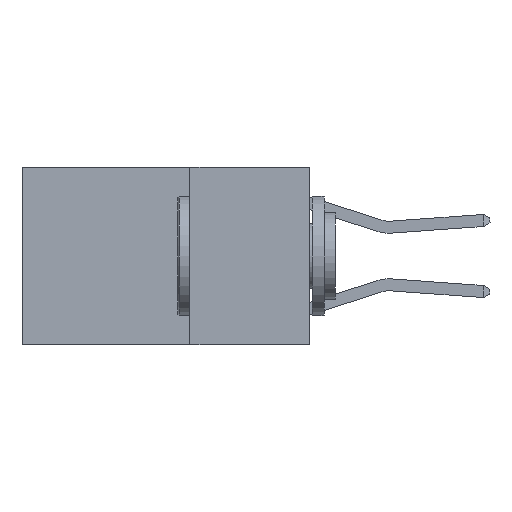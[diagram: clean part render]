
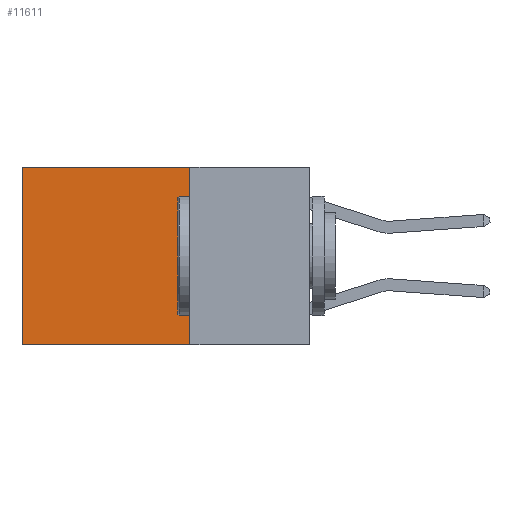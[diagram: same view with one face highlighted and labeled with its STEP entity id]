
A CAD part, left-side view. The second image highlights one B-rep face of the part: STEP entity #11611.
In plain terms, the highlighted planar face has unit normal (-1, 0, 0).
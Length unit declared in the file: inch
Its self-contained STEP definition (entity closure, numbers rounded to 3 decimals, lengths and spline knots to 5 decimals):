
#410 = PLANE ( 'NONE',  #19959 ) ;
#2105 = VERTEX_POINT ( 'NONE', #9692 ) ;
#2933 = DIRECTION ( 'NONE',  ( 0., 0., -1. ) ) ;
#3425 = LINE ( 'NONE', #7947, #3714 ) ;
#3468 = CARTESIAN_POINT ( 'NONE',  ( 0.2625, 0.6, 0. ) ) ;
#3618 = LINE ( 'NONE', #17856, #18739 ) ;
#3714 = VECTOR ( 'NONE', #23025, 39.37008 ) ;
#4959 = CARTESIAN_POINT ( 'NONE',  ( 0.2625, 0.25, 0. ) ) ;
#4989 = ORIENTED_EDGE ( 'NONE', *, *, #12226, .F. ) ;
#5454 = CARTESIAN_POINT ( 'NONE',  ( 0.2625, 0.25, 0. ) ) ;
#6095 = VERTEX_POINT ( 'NONE', #5454 ) ;
#6501 = CARTESIAN_POINT ( 'NONE',  ( 0.2625, 0.25, -0.37 ) ) ;
#7947 = CARTESIAN_POINT ( 'NONE',  ( 0.2625, 0.6, 0. ) ) ;
#8105 = EDGE_CURVE ( 'NONE', #6095, #21910, #3618, .T. ) ;
#8441 = DIRECTION ( 'NONE',  ( 0., 1., 0. ) ) ;
#9320 = VECTOR ( 'NONE', #8441, 39.37008 ) ;
#9692 = CARTESIAN_POINT ( 'NONE',  ( 0.2625, 0.6, -0.37 ) ) ;
#10284 = CARTESIAN_POINT ( 'NONE',  ( 0.2625, 0.25, 0. ) ) ;
#11611 = ADVANCED_FACE ( 'NONE', ( #12530 ), #410, .F. ) ;
#11860 = LINE ( 'NONE', #4959, #13413 ) ;
#12226 = EDGE_CURVE ( 'NONE', #6095, #16497, #11860, .T. ) ;
#12530 = FACE_OUTER_BOUND ( 'NONE', #21019, .T. ) ;
#13123 = EDGE_CURVE ( 'NONE', #21910, #2105, #3425, .T. ) ;
#13413 = VECTOR ( 'NONE', #2933, 39.37008 ) ;
#14027 = DIRECTION ( 'NONE',  ( 0., 0., -1. ) ) ;
#14198 = DIRECTION ( 'NONE',  ( 1., 0., 0. ) ) ;
#16497 = VERTEX_POINT ( 'NONE', #16797 ) ;
#16797 = CARTESIAN_POINT ( 'NONE',  ( 0.2625, 0.25, -0.37 ) ) ;
#17856 = CARTESIAN_POINT ( 'NONE',  ( 0.2625, 0.25, 0. ) ) ;
#18739 = VECTOR ( 'NONE', #23346, 39.37008 ) ;
#19540 = ORIENTED_EDGE ( 'NONE', *, *, #22829, .F. ) ;
#19959 = AXIS2_PLACEMENT_3D ( 'NONE', #10284, #14198, #14027 ) ;
#21019 = EDGE_LOOP ( 'NONE', ( #21455, #19540, #4989, #24924 ) ) ;
#21455 = ORIENTED_EDGE ( 'NONE', *, *, #13123, .T. ) ;
#21910 = VERTEX_POINT ( 'NONE', #3468 ) ;
#22829 = EDGE_CURVE ( 'NONE', #16497, #2105, #24738, .T. ) ;
#23025 = DIRECTION ( 'NONE',  ( 0., 0., -1. ) ) ;
#23346 = DIRECTION ( 'NONE',  ( 0., 1., 0. ) ) ;
#24738 = LINE ( 'NONE', #6501, #9320 ) ;
#24924 = ORIENTED_EDGE ( 'NONE', *, *, #8105, .T. ) ;
